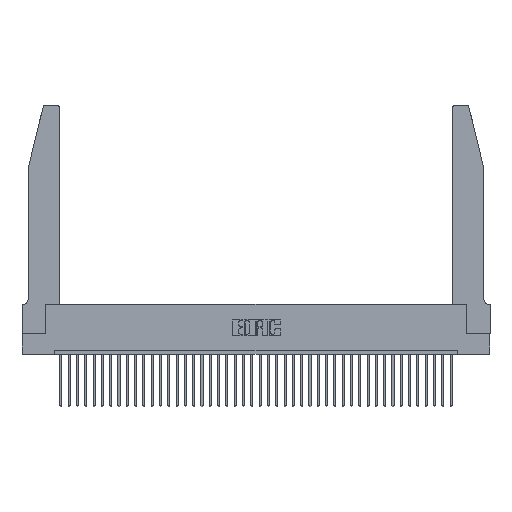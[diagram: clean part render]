
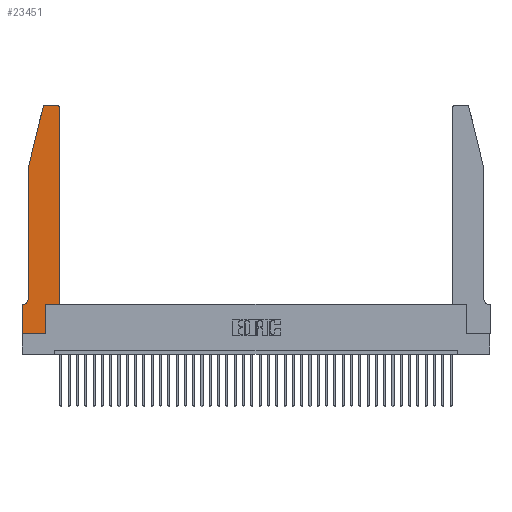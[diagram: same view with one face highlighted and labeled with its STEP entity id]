
A CAD part, top view. The second image highlights one B-rep face of the part: STEP entity #23451.
In plain terms, the highlighted planar face has unit normal (0, 0, 1).
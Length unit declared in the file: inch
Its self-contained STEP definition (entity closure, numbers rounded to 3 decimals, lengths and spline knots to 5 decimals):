
#155 = CARTESIAN_POINT ( 'NONE',  ( 0.0755, 0.35, 0.37 ) ) ;
#263 = EDGE_CURVE ( 'NONE', #10946, #27478, #16585, .T. ) ;
#1187 = ORIENTED_EDGE ( 'NONE', *, *, #4942, .T. ) ;
#1880 = VERTEX_POINT ( 'NONE', #34560 ) ;
#2353 = CARTESIAN_POINT ( 'NONE',  ( 0.2865, 0.35, 0.37 ) ) ;
#2916 = DIRECTION ( 'NONE',  ( -1., 0., 0. ) ) ;
#3000 = DIRECTION ( 'NONE',  ( 1., 0., 0. ) ) ;
#3006 = VERTEX_POINT ( 'NONE', #34616 ) ;
#3799 = CARTESIAN_POINT ( 'NONE',  ( 0.4205, 2.72, 0.37 ) ) ;
#3852 = DIRECTION ( 'NONE',  ( 1., 0., 0. ) ) ;
#3862 = AXIS2_PLACEMENT_3D ( 'NONE', #21985, #12842, #3852 ) ;
#4220 = VECTOR ( 'NONE', #4692, 39.37008 ) ;
#4692 = DIRECTION ( 'NONE',  ( -0.239, -0.971, 0. ) ) ;
#4922 = CARTESIAN_POINT ( 'NONE',  ( 0., 0.35, 0.37 ) ) ;
#4942 = EDGE_CURVE ( 'NONE', #1880, #21017, #27578, .T. ) ;
#5493 = ORIENTED_EDGE ( 'NONE', *, *, #12635, .T. ) ;
#5632 = EDGE_CURVE ( 'NONE', #7689, #10946, #30909, .T. ) ;
#5823 = VECTOR ( 'NONE', #35646, 39.37008 ) ;
#6860 = ORIENTED_EDGE ( 'NONE', *, *, #34240, .T. ) ;
#7495 = ORIENTED_EDGE ( 'NONE', *, *, #10210, .T. ) ;
#7683 = CARTESIAN_POINT ( 'NONE',  ( 0., 0., 0.37 ) ) ;
#7689 = VERTEX_POINT ( 'NONE', #31125 ) ;
#8368 = VECTOR ( 'NONE', #16600, 39.37008 ) ;
#10210 = EDGE_CURVE ( 'NONE', #3006, #36624, #29701, .T. ) ;
#10946 = VERTEX_POINT ( 'NONE', #4922 ) ;
#11035 = VERTEX_POINT ( 'NONE', #40023 ) ;
#11054 = DIRECTION ( 'NONE',  ( -1., 0., 0. ) ) ;
#11061 = VECTOR ( 'NONE', #26771, 39.37008 ) ;
#11355 = PLANE ( 'NONE',  #18222 ) ;
#11683 = CARTESIAN_POINT ( 'NONE',  ( 0.25487, 2.72718, 0.37 ) ) ;
#11708 = EDGE_CURVE ( 'NONE', #22008, #1880, #14199, .T. ) ;
#12007 = CARTESIAN_POINT ( 'NONE',  ( 0., 0., 0.37 ) ) ;
#12173 = ORIENTED_EDGE ( 'NONE', *, *, #263, .T. ) ;
#12317 = CARTESIAN_POINT ( 'NONE',  ( 0.4205, 2.75, 0.37 ) ) ;
#12635 = EDGE_CURVE ( 'NONE', #11035, #35830, #28206, .T. ) ;
#12842 = DIRECTION ( 'NONE',  ( 0., 0., 1. ) ) ;
#12977 = VECTOR ( 'NONE', #3000, 39.37008 ) ;
#13860 = VECTOR ( 'NONE', #40062, 39.37008 ) ;
#13994 = CARTESIAN_POINT ( 'NONE',  ( 0.2605, 2.75, 0.37 ) ) ;
#13999 = VERTEX_POINT ( 'NONE', #33529 ) ;
#14199 = LINE ( 'NONE', #2353, #27383 ) ;
#16585 = LINE ( 'NONE', #7683, #8368 ) ;
#16600 = DIRECTION ( 'NONE',  ( 0., -1., 0. ) ) ;
#16817 = CARTESIAN_POINT ( 'NONE',  ( 0.4505, 0.35, 0.37 ) ) ;
#16829 = DIRECTION ( 'NONE',  ( 0., -1., 0. ) ) ;
#17548 = AXIS2_PLACEMENT_3D ( 'NONE', #30294, #33633, #2916 ) ;
#18222 = AXIS2_PLACEMENT_3D ( 'NONE', #39249, #23727, #20849 ) ;
#18815 = CARTESIAN_POINT ( 'NONE',  ( 0.0755, 0.42, 0.37 ) ) ;
#19438 = VECTOR ( 'NONE', #16829, 39.37008 ) ;
#19886 = EDGE_LOOP ( 'NONE', ( #36667, #5493, #32285, #7495, #32724, #37958, #12173, #38430, #23252, #1187, #6860, #36457 ) ) ;
#19978 = CARTESIAN_POINT ( 'NONE',  ( 0.0755, 2., 0.37 ) ) ;
#20501 = EDGE_CURVE ( 'NONE', #34018, #11035, #22665, .T. ) ;
#20502 = CARTESIAN_POINT ( 'NONE',  ( 0.4505, 0.35, 0.37 ) ) ;
#20607 = CARTESIAN_POINT ( 'NONE',  ( 0., 0., 0.37 ) ) ;
#20849 = DIRECTION ( 'NONE',  ( 1., 0., 0. ) ) ;
#21017 = VERTEX_POINT ( 'NONE', #28392 ) ;
#21185 = VECTOR ( 'NONE', #11054, 39.37008 ) ;
#21310 = EDGE_CURVE ( 'NONE', #35830, #3006, #28402, .T. ) ;
#21985 = CARTESIAN_POINT ( 'NONE',  ( 0.284, 2.72, 0.37 ) ) ;
#22008 = VERTEX_POINT ( 'NONE', #39301 ) ;
#22665 = LINE ( 'NONE', #13994, #21185 ) ;
#22801 = AXIS2_PLACEMENT_3D ( 'NONE', #3799, #31410, #25624 ) ;
#23252 = ORIENTED_EDGE ( 'NONE', *, *, #11708, .T. ) ;
#23451 = ADVANCED_FACE ( 'NONE', ( #31247 ), #11355, .T. ) ;
#23727 = DIRECTION ( 'NONE',  ( 0., 0., 1. ) ) ;
#25624 = DIRECTION ( 'NONE',  ( 1., 0., 0. ) ) ;
#26771 = DIRECTION ( 'NONE',  ( 1., 0., 0. ) ) ;
#27383 = VECTOR ( 'NONE', #36006, 39.37008 ) ;
#27478 = VERTEX_POINT ( 'NONE', #20607 ) ;
#27517 = EDGE_CURVE ( 'NONE', #27478, #22008, #27596, .T. ) ;
#27578 = LINE ( 'NONE', #20502, #11061 ) ;
#27596 = LINE ( 'NONE', #12007, #12977 ) ;
#28206 = CIRCLE ( 'NONE', #3862, 0.03 ) ;
#28392 = CARTESIAN_POINT ( 'NONE',  ( 0.4505, 0.35, 0.37 ) ) ;
#28402 = LINE ( 'NONE', #19978, #4220 ) ;
#29701 = LINE ( 'NONE', #35781, #19438 ) ;
#30294 = CARTESIAN_POINT ( 'NONE',  ( 0.0055, 0.42, 0.37 ) ) ;
#30909 = LINE ( 'NONE', #155, #13860 ) ;
#31125 = CARTESIAN_POINT ( 'NONE',  ( 0.0055, 0.35, 0.37 ) ) ;
#31247 = FACE_OUTER_BOUND ( 'NONE', #19886, .T. ) ;
#31410 = DIRECTION ( 'NONE',  ( 0., 0., 1. ) ) ;
#32066 = CIRCLE ( 'NONE', #22801, 0.03 ) ;
#32285 = ORIENTED_EDGE ( 'NONE', *, *, #21310, .T. ) ;
#32724 = ORIENTED_EDGE ( 'NONE', *, *, #35806, .T. ) ;
#33529 = CARTESIAN_POINT ( 'NONE',  ( 0.4505, 2.72, 0.37 ) ) ;
#33633 = DIRECTION ( 'NONE',  ( 0., 0., -1. ) ) ;
#34018 = VERTEX_POINT ( 'NONE', #12317 ) ;
#34240 = EDGE_CURVE ( 'NONE', #21017, #13999, #39725, .T. ) ;
#34560 = CARTESIAN_POINT ( 'NONE',  ( 0.2865, 0.35, 0.37 ) ) ;
#34616 = CARTESIAN_POINT ( 'NONE',  ( 0.0755, 2., 0.37 ) ) ;
#35646 = DIRECTION ( 'NONE',  ( 0., 1., 0. ) ) ;
#35781 = CARTESIAN_POINT ( 'NONE',  ( 0.0755, 2., 0.37 ) ) ;
#35806 = EDGE_CURVE ( 'NONE', #36624, #7689, #37148, .T. ) ;
#35830 = VERTEX_POINT ( 'NONE', #11683 ) ;
#36006 = DIRECTION ( 'NONE',  ( 0., 1., 0. ) ) ;
#36457 = ORIENTED_EDGE ( 'NONE', *, *, #36698, .T. ) ;
#36624 = VERTEX_POINT ( 'NONE', #18815 ) ;
#36667 = ORIENTED_EDGE ( 'NONE', *, *, #20501, .T. ) ;
#36698 = EDGE_CURVE ( 'NONE', #13999, #34018, #32066, .T. ) ;
#37148 = CIRCLE ( 'NONE', #17548, 0.07 ) ;
#37958 = ORIENTED_EDGE ( 'NONE', *, *, #5632, .T. ) ;
#38430 = ORIENTED_EDGE ( 'NONE', *, *, #27517, .T. ) ;
#39249 = CARTESIAN_POINT ( 'NONE',  ( 0., 0.35, 0.37 ) ) ;
#39301 = CARTESIAN_POINT ( 'NONE',  ( 0.2865, 0., 0.37 ) ) ;
#39725 = LINE ( 'NONE', #16817, #5823 ) ;
#40023 = CARTESIAN_POINT ( 'NONE',  ( 0.284, 2.75, 0.37 ) ) ;
#40062 = DIRECTION ( 'NONE',  ( -1., 0., 0. ) ) ;
